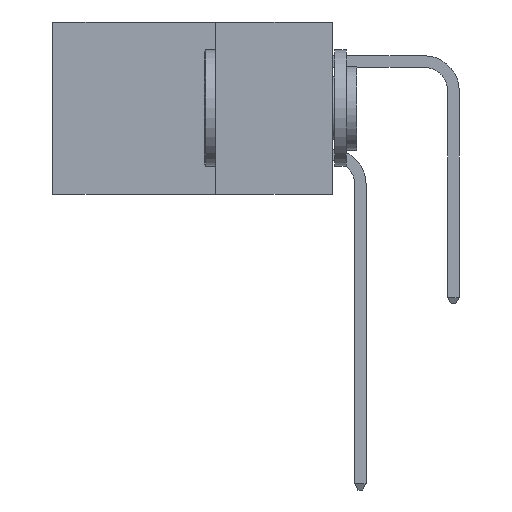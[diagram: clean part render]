
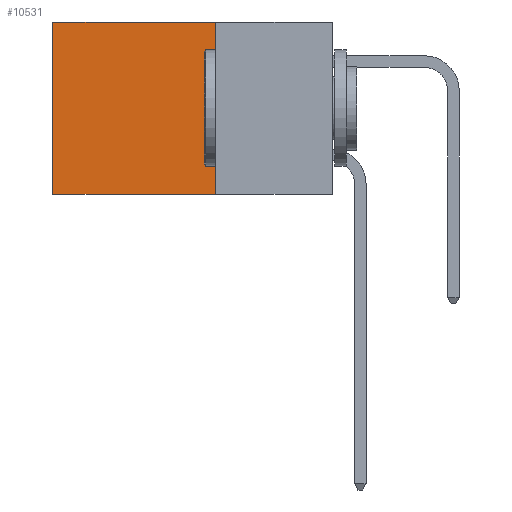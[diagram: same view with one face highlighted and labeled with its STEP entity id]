
A CAD part, left-side view. The second image highlights one B-rep face of the part: STEP entity #10531.
In plain terms, the highlighted planar face has unit normal (-1, 0, 0).
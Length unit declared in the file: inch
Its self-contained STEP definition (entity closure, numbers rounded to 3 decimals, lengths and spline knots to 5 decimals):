
#656 = ORIENTED_EDGE ( 'NONE', *, *, #939, .F. ) ;
#735 = CARTESIAN_POINT ( 'NONE',  ( 0.2615, 0.25, -0.37 ) ) ;
#939 = EDGE_CURVE ( 'NONE', #5551, #2979, #5426, .T. ) ;
#995 = ORIENTED_EDGE ( 'NONE', *, *, #2146, .T. ) ;
#1978 = LINE ( 'NONE', #13548, #4889 ) ;
#2103 = EDGE_CURVE ( 'NONE', #2979, #5568, #10948, .T. ) ;
#2146 = EDGE_CURVE ( 'NONE', #5551, #13842, #13488, .T. ) ;
#2220 = DIRECTION ( 'NONE',  ( 0., 1., 0. ) ) ;
#2443 = CARTESIAN_POINT ( 'NONE',  ( 0.2615, 0.6, 0. ) ) ;
#2636 = CARTESIAN_POINT ( 'NONE',  ( 0.2615, 0.6, -0.37 ) ) ;
#2848 = EDGE_CURVE ( 'NONE', #13842, #5568, #1978, .T. ) ;
#2979 = VERTEX_POINT ( 'NONE', #735 ) ;
#4674 = AXIS2_PLACEMENT_3D ( 'NONE', #6105, #13615, #7202 ) ;
#4889 = VECTOR ( 'NONE', #7141, 39.37008 ) ;
#5220 = VECTOR ( 'NONE', #2220, 39.37008 ) ;
#5277 = CARTESIAN_POINT ( 'NONE',  ( 0.2615, 0.25, 0. ) ) ;
#5426 = LINE ( 'NONE', #7087, #10484 ) ;
#5551 = VERTEX_POINT ( 'NONE', #10175 ) ;
#5568 = VERTEX_POINT ( 'NONE', #2636 ) ;
#6105 = CARTESIAN_POINT ( 'NONE',  ( 0.2615, 0.25, -0.37 ) ) ;
#6287 = EDGE_LOOP ( 'NONE', ( #8689, #9044, #656, #995 ) ) ;
#6511 = DIRECTION ( 'NONE',  ( 0., 1., 0. ) ) ;
#7087 = CARTESIAN_POINT ( 'NONE',  ( 0.2615, 0.25, -0.37 ) ) ;
#7141 = DIRECTION ( 'NONE',  ( 0., 0., -1. ) ) ;
#7202 = DIRECTION ( 'NONE',  ( 0., 0., -1. ) ) ;
#7444 = VECTOR ( 'NONE', #6511, 39.37008 ) ;
#8272 = DIRECTION ( 'NONE',  ( 0., 0., -1. ) ) ;
#8689 = ORIENTED_EDGE ( 'NONE', *, *, #2848, .T. ) ;
#9044 = ORIENTED_EDGE ( 'NONE', *, *, #2103, .F. ) ;
#10175 = CARTESIAN_POINT ( 'NONE',  ( 0.2615, 0.25, 0. ) ) ;
#10484 = VECTOR ( 'NONE', #8272, 39.37008 ) ;
#10531 = ADVANCED_FACE ( 'NONE', ( #10606 ), #12538, .F. ) ;
#10606 = FACE_OUTER_BOUND ( 'NONE', #6287, .T. ) ;
#10948 = LINE ( 'NONE', #11148, #5220 ) ;
#11148 = CARTESIAN_POINT ( 'NONE',  ( 0.2615, 0.25, -0.37 ) ) ;
#12538 = PLANE ( 'NONE',  #4674 ) ;
#13488 = LINE ( 'NONE', #5277, #7444 ) ;
#13548 = CARTESIAN_POINT ( 'NONE',  ( 0.2615, 0.6, -0.37 ) ) ;
#13615 = DIRECTION ( 'NONE',  ( 1., 0., 0. ) ) ;
#13842 = VERTEX_POINT ( 'NONE', #2443 ) ;
